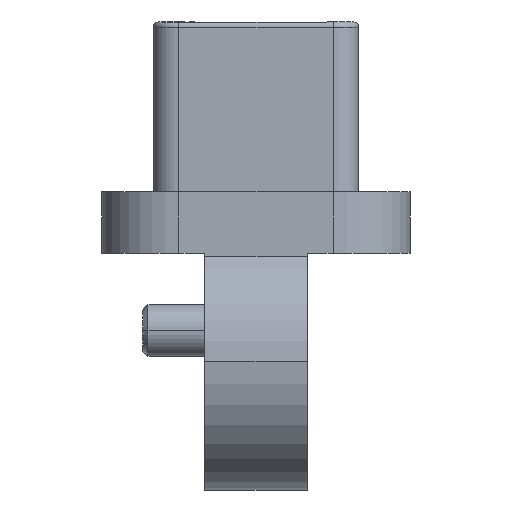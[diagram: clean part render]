
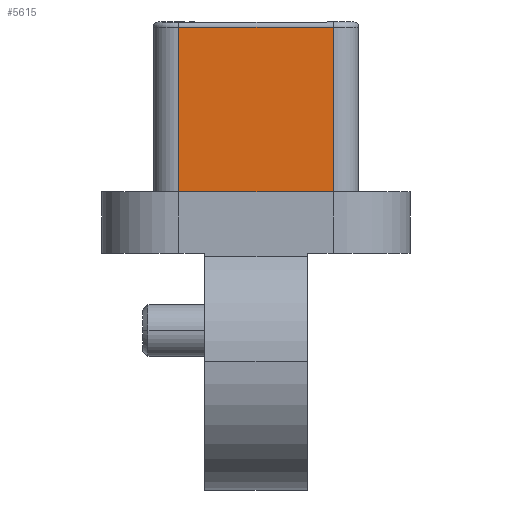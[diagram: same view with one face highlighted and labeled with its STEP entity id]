
A CAD part, left-side view. The second image highlights one B-rep face of the part: STEP entity #5615.
In plain terms, the highlighted planar face has unit normal (-1, 0, 0).
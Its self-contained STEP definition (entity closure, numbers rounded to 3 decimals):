
#403 = VECTOR ( 'NONE', #7480, 1000. ) ;
#466 = DIRECTION ( 'NONE',  ( 0., 0., -1. ) ) ;
#688 = EDGE_CURVE ( 'NONE', #1839, #4002, #3405, .T. ) ;
#838 = EDGE_LOOP ( 'NONE', ( #5604, #3769, #3539, #4014 ) ) ;
#1115 = EDGE_CURVE ( 'NONE', #5356, #2638, #1193, .T. ) ;
#1193 = LINE ( 'NONE', #3531, #3136 ) ;
#1685 = DIRECTION ( 'NONE',  ( 0., 1., 0. ) ) ;
#1839 = VERTEX_POINT ( 'NONE', #4143 ) ;
#2077 = DIRECTION ( 'NONE',  ( 1., 0., 0. ) ) ;
#2453 = EDGE_CURVE ( 'NONE', #4002, #5356, #2763, .T. ) ;
#2638 = VERTEX_POINT ( 'NONE', #3015 ) ;
#2650 = FACE_OUTER_BOUND ( 'NONE', #838, .T. ) ;
#2763 = LINE ( 'NONE', #5112, #403 ) ;
#2905 = VECTOR ( 'NONE', #466, 1000. ) ;
#3015 = CARTESIAN_POINT ( 'NONE',  ( -8.45, -1.5, -0.1 ) ) ;
#3023 = AXIS2_PLACEMENT_3D ( 'NONE', #7363, #2077, #4417 ) ;
#3136 = VECTOR ( 'NONE', #5919, 1000. ) ;
#3405 = LINE ( 'NONE', #5784, #2905 ) ;
#3531 = CARTESIAN_POINT ( 'NONE',  ( -8.45, -1.5, -3.3 ) ) ;
#3539 = ORIENTED_EDGE ( 'NONE', *, *, #1115, .T. ) ;
#3769 = ORIENTED_EDGE ( 'NONE', *, *, #2453, .T. ) ;
#4002 = VERTEX_POINT ( 'NONE', #4225 ) ;
#4014 = ORIENTED_EDGE ( 'NONE', *, *, #4607, .T. ) ;
#4051 = VECTOR ( 'NONE', #1685, 1000. ) ;
#4143 = CARTESIAN_POINT ( 'NONE',  ( -8.45, 1.5, -0.1 ) ) ;
#4225 = CARTESIAN_POINT ( 'NONE',  ( -8.45, 1.5, -3.3 ) ) ;
#4417 = DIRECTION ( 'NONE',  ( 0., 1., 0. ) ) ;
#4593 = LINE ( 'NONE', #6982, #4051 ) ;
#4607 = EDGE_CURVE ( 'NONE', #2638, #1839, #4593, .T. ) ;
#4994 = PLANE ( 'NONE',  #3023 ) ;
#5112 = CARTESIAN_POINT ( 'NONE',  ( -8.45, 1.5, -3.3 ) ) ;
#5356 = VERTEX_POINT ( 'NONE', #6356 ) ;
#5604 = ORIENTED_EDGE ( 'NONE', *, *, #688, .T. ) ;
#5615 = ADVANCED_FACE ( 'NONE', ( #2650 ), #4994, .F. ) ;
#5784 = CARTESIAN_POINT ( 'NONE',  ( -8.45, 1.5, -0.1 ) ) ;
#5919 = DIRECTION ( 'NONE',  ( 0., 0., 1. ) ) ;
#6356 = CARTESIAN_POINT ( 'NONE',  ( -8.45, -1.5, -3.3 ) ) ;
#6982 = CARTESIAN_POINT ( 'NONE',  ( -8.45, -1.5, -0.1 ) ) ;
#7363 = CARTESIAN_POINT ( 'NONE',  ( -8.45, 0., -1.7 ) ) ;
#7480 = DIRECTION ( 'NONE',  ( 0., -1., 0. ) ) ;
